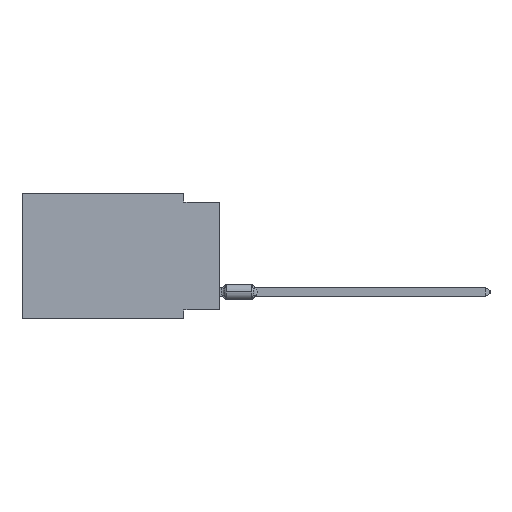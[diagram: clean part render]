
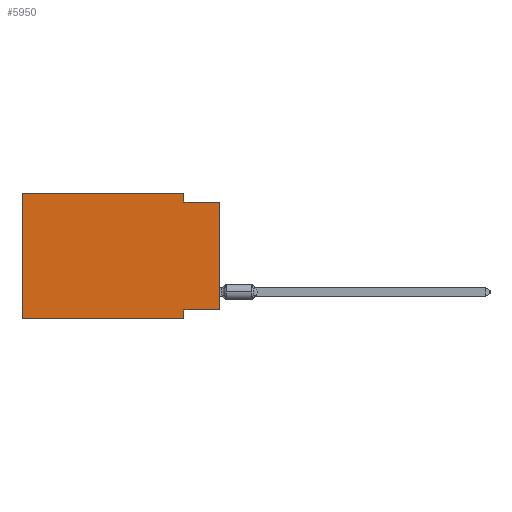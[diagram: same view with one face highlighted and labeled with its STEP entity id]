
A CAD part, left-side view. The second image highlights one B-rep face of the part: STEP entity #5950.
In plain terms, the highlighted planar face has unit normal (-1, 0, 0).
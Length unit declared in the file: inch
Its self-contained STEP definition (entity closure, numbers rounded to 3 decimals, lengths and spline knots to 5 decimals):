
#591 = PLANE ( 'NONE',  #32462 ) ;
#944 = CARTESIAN_POINT ( 'NONE',  ( 0., 0.1, -0.325 ) ) ;
#1173 = ORIENTED_EDGE ( 'NONE', *, *, #47000, .F. ) ;
#3046 = ORIENTED_EDGE ( 'NONE', *, *, #60564, .F. ) ;
#5201 = VERTEX_POINT ( 'NONE', #69752 ) ;
#5950 = ADVANCED_FACE ( 'NONE', ( #54134 ), #591, .F. ) ;
#6557 = DIRECTION ( 'NONE',  ( 1., 0., 0. ) ) ;
#7724 = VECTOR ( 'NONE', #16046, 39.37008 ) ;
#10330 = CARTESIAN_POINT ( 'NONE',  ( 0., 0., -0.025 ) ) ;
#11579 = CARTESIAN_POINT ( 'NONE',  ( 0., 0.55, -0.35 ) ) ;
#16046 = DIRECTION ( 'NONE',  ( 0., 1., 0. ) ) ;
#16747 = ORIENTED_EDGE ( 'NONE', *, *, #28103, .F. ) ;
#17261 = ORIENTED_EDGE ( 'NONE', *, *, #61693, .F. ) ;
#17345 = CARTESIAN_POINT ( 'NONE',  ( 0., 0.1, -0.35 ) ) ;
#18680 = CARTESIAN_POINT ( 'NONE',  ( 0., 0., -0.325 ) ) ;
#18699 = CARTESIAN_POINT ( 'NONE',  ( 0., 0., -0.325 ) ) ;
#19140 = VECTOR ( 'NONE', #76400, 39.37008 ) ;
#19952 = LINE ( 'NONE', #55635, #21840 ) ;
#20779 = EDGE_LOOP ( 'NONE', ( #63404, #3046, #71206, #17261, #69646, #52641, #1173, #16747 ) ) ;
#20963 = VERTEX_POINT ( 'NONE', #944 ) ;
#21840 = VECTOR ( 'NONE', #57200, 39.37008 ) ;
#23021 = VERTEX_POINT ( 'NONE', #10330 ) ;
#24243 = LINE ( 'NONE', #18680, #7724 ) ;
#24516 = DIRECTION ( 'NONE',  ( 0., 0., 1. ) ) ;
#26470 = EDGE_CURVE ( 'NONE', #38335, #75288, #36559, .T. ) ;
#28103 = EDGE_CURVE ( 'NONE', #64376, #20963, #24243, .T. ) ;
#32462 = AXIS2_PLACEMENT_3D ( 'NONE', #55710, #6557, #72393 ) ;
#32908 = EDGE_CURVE ( 'NONE', #38335, #5201, #35271, .T. ) ;
#33406 = LINE ( 'NONE', #45272, #45828 ) ;
#35271 = LINE ( 'NONE', #55029, #69364 ) ;
#35857 = VECTOR ( 'NONE', #72986, 39.37008 ) ;
#36396 = DIRECTION ( 'NONE',  ( 0., 0., -1. ) ) ;
#36559 = LINE ( 'NONE', #11579, #42988 ) ;
#38335 = VERTEX_POINT ( 'NONE', #54463 ) ;
#38642 = EDGE_CURVE ( 'NONE', #64376, #23021, #53373, .T. ) ;
#42988 = VECTOR ( 'NONE', #53210, 39.37008 ) ;
#43237 = CARTESIAN_POINT ( 'NONE',  ( 0., 0.1, 0. ) ) ;
#44392 = EDGE_CURVE ( 'NONE', #66019, #61400, #78142, .T. ) ;
#45272 = CARTESIAN_POINT ( 'NONE',  ( 0., 0., -0.025 ) ) ;
#45828 = VECTOR ( 'NONE', #70651, 39.37008 ) ;
#47000 = EDGE_CURVE ( 'NONE', #20963, #75288, #64670, .T. ) ;
#49888 = CARTESIAN_POINT ( 'NONE',  ( 0., 0.1, 0. ) ) ;
#52641 = ORIENTED_EDGE ( 'NONE', *, *, #26470, .T. ) ;
#53210 = DIRECTION ( 'NONE',  ( 0., -1., 0. ) ) ;
#53373 = LINE ( 'NONE', #71622, #19140 ) ;
#53767 = VECTOR ( 'NONE', #36396, 39.37008 ) ;
#54134 = FACE_OUTER_BOUND ( 'NONE', #20779, .T. ) ;
#54463 = CARTESIAN_POINT ( 'NONE',  ( 0., 0.55, -0.35 ) ) ;
#55029 = CARTESIAN_POINT ( 'NONE',  ( 0., 0.55, 0. ) ) ;
#55635 = CARTESIAN_POINT ( 'NONE',  ( 0., 0.55, 0. ) ) ;
#55710 = CARTESIAN_POINT ( 'NONE',  ( 0., 0.55, 0. ) ) ;
#57200 = DIRECTION ( 'NONE',  ( 0., -1., 0. ) ) ;
#60564 = EDGE_CURVE ( 'NONE', #61400, #23021, #33406, .T. ) ;
#61400 = VERTEX_POINT ( 'NONE', #75930 ) ;
#61693 = EDGE_CURVE ( 'NONE', #5201, #66019, #19952, .T. ) ;
#63404 = ORIENTED_EDGE ( 'NONE', *, *, #38642, .T. ) ;
#64376 = VERTEX_POINT ( 'NONE', #18699 ) ;
#64670 = LINE ( 'NONE', #76962, #53767 ) ;
#66019 = VERTEX_POINT ( 'NONE', #49888 ) ;
#69364 = VECTOR ( 'NONE', #24516, 39.37008 ) ;
#69646 = ORIENTED_EDGE ( 'NONE', *, *, #32908, .F. ) ;
#69752 = CARTESIAN_POINT ( 'NONE',  ( 0., 0.55, 0. ) ) ;
#70651 = DIRECTION ( 'NONE',  ( 0., -1., 0. ) ) ;
#71206 = ORIENTED_EDGE ( 'NONE', *, *, #44392, .F. ) ;
#71622 = CARTESIAN_POINT ( 'NONE',  ( 0., 0., 0. ) ) ;
#72393 = DIRECTION ( 'NONE',  ( 0., 0., -1. ) ) ;
#72986 = DIRECTION ( 'NONE',  ( 0., 0., -1. ) ) ;
#75288 = VERTEX_POINT ( 'NONE', #17345 ) ;
#75930 = CARTESIAN_POINT ( 'NONE',  ( 0., 0.1, -0.025 ) ) ;
#76400 = DIRECTION ( 'NONE',  ( 0., 0., 1. ) ) ;
#76962 = CARTESIAN_POINT ( 'NONE',  ( 0., 0.1, -0.35 ) ) ;
#78142 = LINE ( 'NONE', #43237, #35857 ) ;
